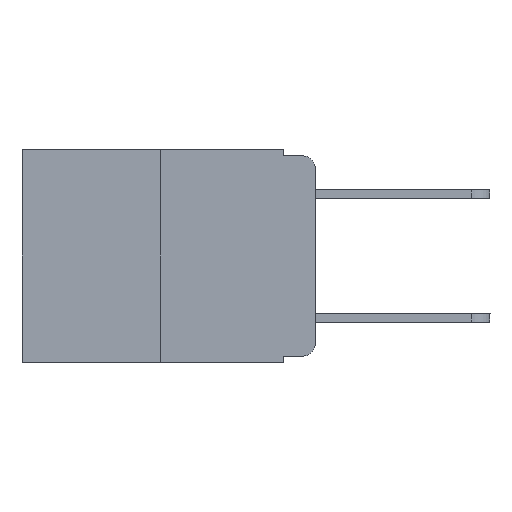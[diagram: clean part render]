
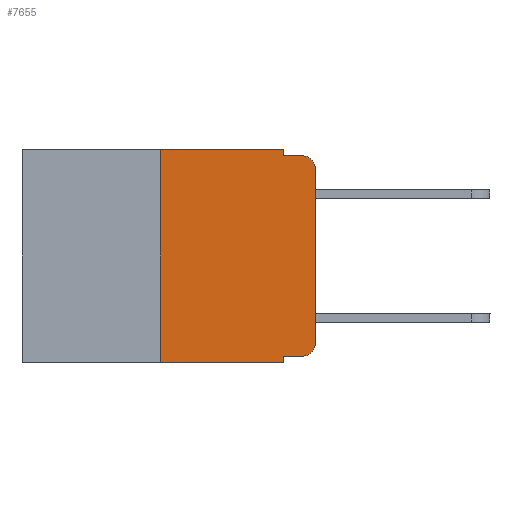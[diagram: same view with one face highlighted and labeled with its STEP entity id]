
A CAD part, left-side view. The second image highlights one B-rep face of the part: STEP entity #7655.
In plain terms, the highlighted planar face has unit normal (-1, 0, 0).
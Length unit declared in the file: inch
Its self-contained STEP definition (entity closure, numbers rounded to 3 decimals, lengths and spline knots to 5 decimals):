
#12 = EDGE_CURVE ( 'NONE', #5273, #10007, #19, .T. ) ;
#19 = LINE ( 'NONE', #4286, #7422 ) ;
#74 = VECTOR ( 'NONE', #9947, 39.37008 ) ;
#92 = ORIENTED_EDGE ( 'NONE', *, *, #6991, .F. ) ;
#116 = CARTESIAN_POINT ( 'NONE',  ( 0., 0.051, -0.333 ) ) ;
#129 = DIRECTION ( 'NONE',  ( 0., 0., -1. ) ) ;
#237 = VERTEX_POINT ( 'NONE', #3996 ) ;
#251 = LINE ( 'NONE', #2328, #3477 ) ;
#265 = CARTESIAN_POINT ( 'NONE',  ( 0., 0.02, -0.333 ) ) ;
#917 = EDGE_CURVE ( 'NONE', #2004, #1392, #5258, .T. ) ;
#947 = DIRECTION ( 'NONE',  ( 1., 0., 0. ) ) ;
#974 = CARTESIAN_POINT ( 'NONE',  ( 0., 0.25, 0. ) ) ;
#1392 = VERTEX_POINT ( 'NONE', #265 ) ;
#1524 = CARTESIAN_POINT ( 'NONE',  ( 0., 0.02, -0.03 ) ) ;
#1632 = CARTESIAN_POINT ( 'NONE',  ( 0., 0.473, -0.343 ) ) ;
#1758 = EDGE_CURVE ( 'NONE', #6067, #237, #7134, .T. ) ;
#1863 = EDGE_CURVE ( 'NONE', #2714, #2544, #7006, .T. ) ;
#2004 = VERTEX_POINT ( 'NONE', #8742 ) ;
#2157 = AXIS2_PLACEMENT_3D ( 'NONE', #5931, #947, #4199 ) ;
#2235 = VECTOR ( 'NONE', #129, 39.37008 ) ;
#2328 = CARTESIAN_POINT ( 'NONE',  ( 0., 0.051, 0. ) ) ;
#2458 = DIRECTION ( 'NONE',  ( 0., -1., 0. ) ) ;
#2544 = VERTEX_POINT ( 'NONE', #7062 ) ;
#2615 = CARTESIAN_POINT ( 'NONE',  ( 0., 0.02, -0.01 ) ) ;
#2714 = VERTEX_POINT ( 'NONE', #4975 ) ;
#2934 = CARTESIAN_POINT ( 'NONE',  ( 0., 0.051, 0. ) ) ;
#3197 = AXIS2_PLACEMENT_3D ( 'NONE', #1524, #4770, #6523 ) ;
#3477 = VECTOR ( 'NONE', #8864, 39.37008 ) ;
#3481 = DIRECTION ( 'NONE',  ( 0., -1., 0. ) ) ;
#3545 = ORIENTED_EDGE ( 'NONE', *, *, #917, .T. ) ;
#3683 = FACE_OUTER_BOUND ( 'NONE', #5351, .T. ) ;
#3692 = DIRECTION ( 'NONE',  ( 0., 0., -1. ) ) ;
#3730 = VERTEX_POINT ( 'NONE', #2615 ) ;
#3833 = EDGE_CURVE ( 'NONE', #2004, #237, #8673, .T. ) ;
#3996 = CARTESIAN_POINT ( 'NONE',  ( 0., 0.051, -0.343 ) ) ;
#4199 = DIRECTION ( 'NONE',  ( 0., 0., -1. ) ) ;
#4286 = CARTESIAN_POINT ( 'NONE',  ( 0., 0.473, 0. ) ) ;
#4667 = ORIENTED_EDGE ( 'NONE', *, *, #6119, .F. ) ;
#4770 = DIRECTION ( 'NONE',  ( -1., 0., 0. ) ) ;
#4885 = EDGE_CURVE ( 'NONE', #6127, #3730, #6708, .T. ) ;
#4975 = CARTESIAN_POINT ( 'NONE',  ( 0., 0., -0.313 ) ) ;
#5166 = CARTESIAN_POINT ( 'NONE',  ( 0., 0.051, 0. ) ) ;
#5258 = LINE ( 'NONE', #116, #7648 ) ;
#5273 = VERTEX_POINT ( 'NONE', #8353 ) ;
#5351 = EDGE_LOOP ( 'NONE', ( #6589, #5652, #9976, #4667, #9666, #92, #6142, #8879, #3545, #6817 ) ) ;
#5652 = ORIENTED_EDGE ( 'NONE', *, *, #8663, .T. ) ;
#5846 = PLANE ( 'NONE',  #2157 ) ;
#5931 = CARTESIAN_POINT ( 'NONE',  ( 0., 0.473, 0. ) ) ;
#5977 = CIRCLE ( 'NONE', #8322, 0.02 ) ;
#6067 = VERTEX_POINT ( 'NONE', #7873 ) ;
#6119 = EDGE_CURVE ( 'NONE', #10007, #6127, #251, .T. ) ;
#6127 = VERTEX_POINT ( 'NONE', #6504 ) ;
#6142 = ORIENTED_EDGE ( 'NONE', *, *, #1758, .T. ) ;
#6460 = CIRCLE ( 'NONE', #3197, 0.02 ) ;
#6504 = CARTESIAN_POINT ( 'NONE',  ( 0., 0.051, -0.01 ) ) ;
#6523 = DIRECTION ( 'NONE',  ( 0., 0., -1. ) ) ;
#6589 = ORIENTED_EDGE ( 'NONE', *, *, #1863, .T. ) ;
#6708 = LINE ( 'NONE', #9050, #8538 ) ;
#6817 = ORIENTED_EDGE ( 'NONE', *, *, #7737, .T. ) ;
#6901 = DIRECTION ( 'NONE',  ( -1., 0., 0. ) ) ;
#6991 = EDGE_CURVE ( 'NONE', #6067, #5273, #9746, .T. ) ;
#7006 = LINE ( 'NONE', #10523, #9366 ) ;
#7062 = CARTESIAN_POINT ( 'NONE',  ( 0., 0., -0.03 ) ) ;
#7134 = LINE ( 'NONE', #1632, #7508 ) ;
#7358 = DIRECTION ( 'NONE',  ( 0., -1., 0. ) ) ;
#7422 = VECTOR ( 'NONE', #7500, 39.37008 ) ;
#7500 = DIRECTION ( 'NONE',  ( 0., -1., 0. ) ) ;
#7508 = VECTOR ( 'NONE', #2458, 39.37008 ) ;
#7648 = VECTOR ( 'NONE', #7358, 39.37008 ) ;
#7655 = ADVANCED_FACE ( 'NONE', ( #3683 ), #5846, .F. ) ;
#7737 = EDGE_CURVE ( 'NONE', #1392, #2714, #5977, .T. ) ;
#7873 = CARTESIAN_POINT ( 'NONE',  ( 0., 0.25, -0.343 ) ) ;
#8322 = AXIS2_PLACEMENT_3D ( 'NONE', #10014, #6901, #3692 ) ;
#8353 = CARTESIAN_POINT ( 'NONE',  ( 0., 0.25, 0. ) ) ;
#8538 = VECTOR ( 'NONE', #3481, 39.37008 ) ;
#8663 = EDGE_CURVE ( 'NONE', #2544, #3730, #6460, .T. ) ;
#8673 = LINE ( 'NONE', #5166, #2235 ) ;
#8742 = CARTESIAN_POINT ( 'NONE',  ( 0., 0.051, -0.333 ) ) ;
#8864 = DIRECTION ( 'NONE',  ( 0., 0., -1. ) ) ;
#8879 = ORIENTED_EDGE ( 'NONE', *, *, #3833, .F. ) ;
#9050 = CARTESIAN_POINT ( 'NONE',  ( 0., 0.051, -0.01 ) ) ;
#9366 = VECTOR ( 'NONE', #9582, 39.37008 ) ;
#9582 = DIRECTION ( 'NONE',  ( 0., 0., 1. ) ) ;
#9666 = ORIENTED_EDGE ( 'NONE', *, *, #12, .F. ) ;
#9746 = LINE ( 'NONE', #974, #74 ) ;
#9947 = DIRECTION ( 'NONE',  ( 0., 0., 1. ) ) ;
#9976 = ORIENTED_EDGE ( 'NONE', *, *, #4885, .F. ) ;
#10007 = VERTEX_POINT ( 'NONE', #2934 ) ;
#10014 = CARTESIAN_POINT ( 'NONE',  ( 0., 0.02, -0.313 ) ) ;
#10523 = CARTESIAN_POINT ( 'NONE',  ( 0., 0., 0. ) ) ;
